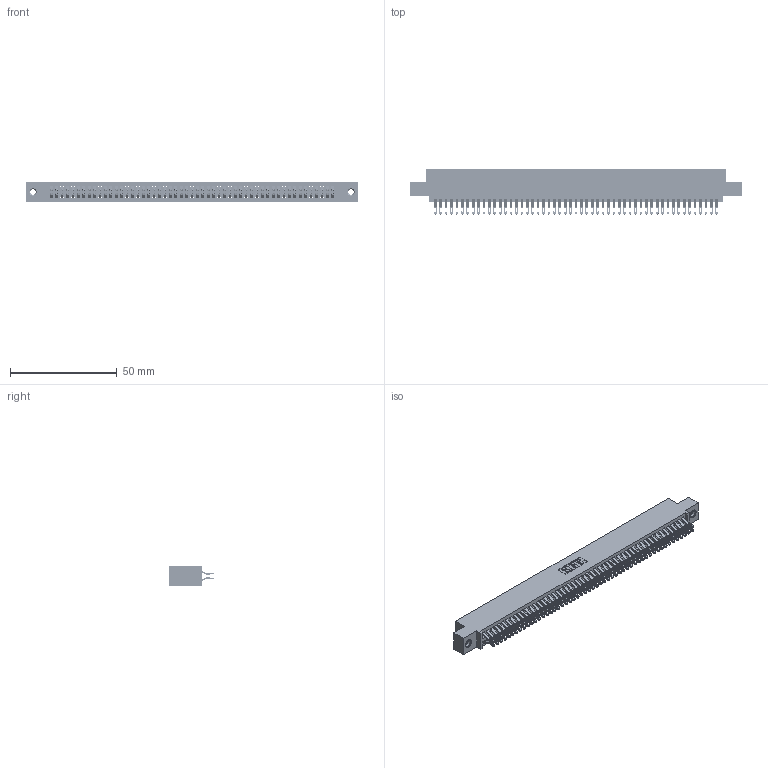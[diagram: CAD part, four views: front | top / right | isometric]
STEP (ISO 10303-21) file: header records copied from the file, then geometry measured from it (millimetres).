
FILE_DESCRIPTION (( 'STEP AP203' ), '1' );
FILE_NAME ('345-106-555-507.STEP', '2019-11-03T17:03:37', ( '' ), ( '' ), 'SwSTEP 2.0', 'SolidWorks 2016', '' );
FILE_SCHEMA (( 'CONFIG_CONTROL_DESIGN' ));
Length unit declared in the file: inch
Products named in the file (4): 345-250-001_345-250-005-103; 345 Part_0.110 Offset - 0.156 Dia-TI; 345-106-555-507; 345-292-001_555 Tail
Assembly tree (109 placements, depth 2):
  345-106-555-507
    345 Part_0.110 Offset - 0.156 Dia-TI
    345-292-001_555 Tail  x106
    345-250-001_345-250-005-103  x2
Bounding box: 155.83 x 21.13 x 9.4 mm (x, y, z)
Volume: 15460.1 mm3; surface area: 24255.7 mm2
Topology: 109 solids, 109 shells, 6126 faces, 19251 edges, 12826 vertices
Faces by surface type: plane 3402, cylinder 2708, cone 12, torus 4
Entity records: 41748 total; most frequent: CARTESIAN_POINT 7005, ORIENTED_EDGE 6902, DIRECTION 6157, EDGE_CURVE 3451, LINE 3067, VECTOR 3067, VERTEX_POINT 2296, AXIS2_PLACEMENT_3D 1545
